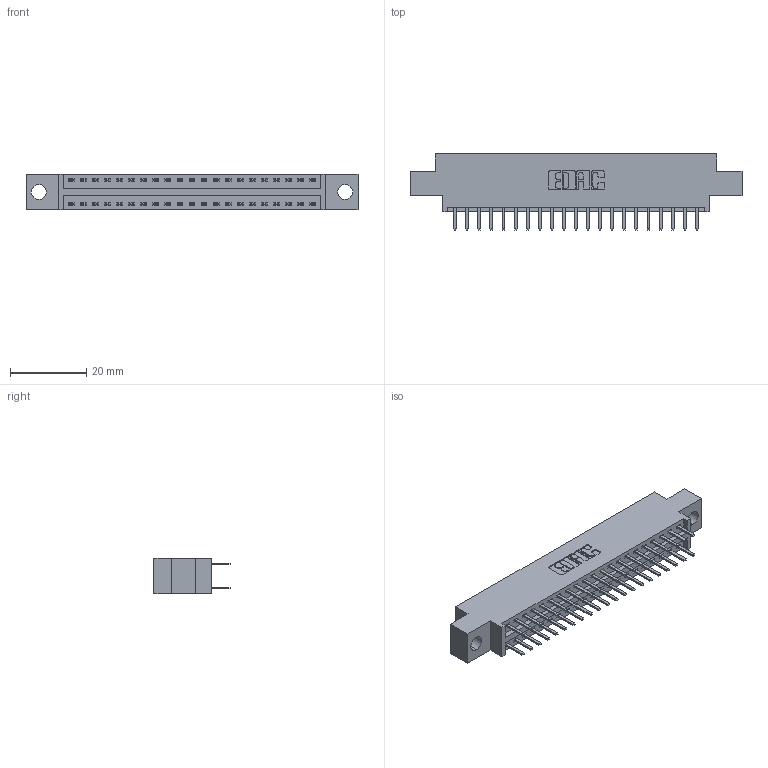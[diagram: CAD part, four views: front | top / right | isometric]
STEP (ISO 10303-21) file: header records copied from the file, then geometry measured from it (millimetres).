
FILE_DESCRIPTION (( 'STEP AP203' ), '1' );
FILE_NAME ('346-042-520-804.STEP', '2022-05-20T03:42:23', ( '' ), ( '' ), 'SwSTEP 2.0', 'SolidWorks 2020', '' );
FILE_SCHEMA (( 'CONFIG_CONTROL_DESIGN' ));
Length unit declared in the file: inch
Products named in the file (3): 346 Part_0.170 Offset - 0.156 Dia-TH; 345-292-001_345-293-120; 346-042-520-804
Assembly tree (43 placements, depth 2):
  346-042-520-804
    346 Part_0.170 Offset - 0.156 Dia-TH
    345-292-001_345-293-120  x42
Bounding box: 87.25 x 20.02 x 9.4 mm (x, y, z)
Volume: 8065.7 mm3; surface area: 10741.1 mm2
Topology: 43 solids, 43 shells, 2492 faces, 7223 edges, 4702 vertices
Faces by surface type: plane 1648, cylinder 844
Entity records: 17197 total; most frequent: CARTESIAN_POINT 2882, ORIENTED_EDGE 2802, DIRECTION 2577, EDGE_CURVE 1401, VECTOR 1181, LINE 1181, VERTEX_POINT 930, AXIS2_PLACEMENT_3D 698
